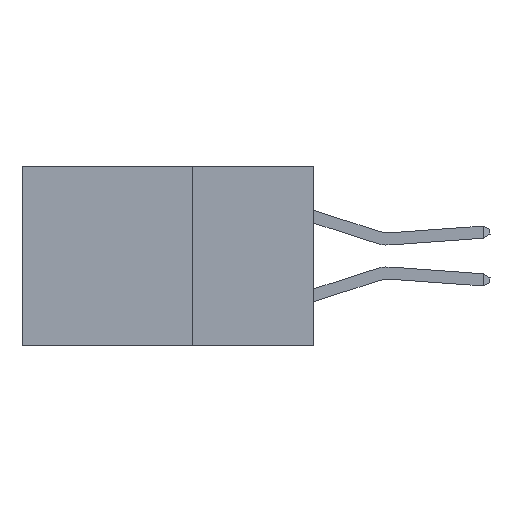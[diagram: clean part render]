
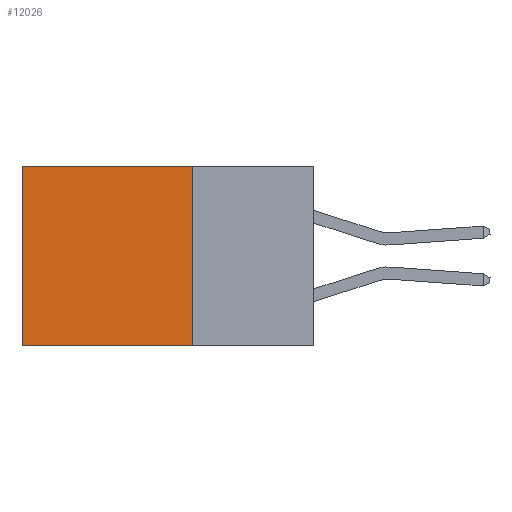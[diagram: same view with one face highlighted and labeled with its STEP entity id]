
A CAD part, left-side view. The second image highlights one B-rep face of the part: STEP entity #12026.
In plain terms, the highlighted planar face has unit normal (-1, 0, 0).
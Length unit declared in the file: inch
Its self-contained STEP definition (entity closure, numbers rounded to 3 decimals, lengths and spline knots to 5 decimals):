
#648 = AXIS2_PLACEMENT_3D ( 'NONE', #25661, #12626, #22278 ) ;
#1149 = VECTOR ( 'NONE', #2713, 39.37008 ) ;
#1549 = VERTEX_POINT ( 'NONE', #24139 ) ;
#2001 = CARTESIAN_POINT ( 'NONE',  ( 0.2875, 0.25, -0.37 ) ) ;
#2713 = DIRECTION ( 'NONE',  ( 0., 0., -1. ) ) ;
#3283 = CARTESIAN_POINT ( 'NONE',  ( 0.2875, 0.6, 0. ) ) ;
#3468 = DIRECTION ( 'NONE',  ( 0., 1., 0. ) ) ;
#3616 = EDGE_CURVE ( 'NONE', #1549, #25692, #10830, .T. ) ;
#3945 = VERTEX_POINT ( 'NONE', #22671 ) ;
#3960 = PLANE ( 'NONE',  #648 ) ;
#3964 = ORIENTED_EDGE ( 'NONE', *, *, #16884, .F. ) ;
#6012 = DIRECTION ( 'NONE',  ( 0., 1., 0. ) ) ;
#7553 = DIRECTION ( 'NONE',  ( 0., 0., -1. ) ) ;
#8371 = LINE ( 'NONE', #25355, #23628 ) ;
#8991 = EDGE_LOOP ( 'NONE', ( #12165, #3964, #16511, #22000 ) ) ;
#10705 = CARTESIAN_POINT ( 'NONE',  ( 0.2875, 0.6, -0.37 ) ) ;
#10830 = LINE ( 'NONE', #3283, #15815 ) ;
#12026 = ADVANCED_FACE ( 'NONE', ( #14006 ), #3960, .F. ) ;
#12165 = ORIENTED_EDGE ( 'NONE', *, *, #3616, .T. ) ;
#12626 = DIRECTION ( 'NONE',  ( 1., 0., 0. ) ) ;
#14006 = FACE_OUTER_BOUND ( 'NONE', #8991, .T. ) ;
#14038 = VERTEX_POINT ( 'NONE', #24936 ) ;
#15815 = VECTOR ( 'NONE', #7553, 39.37008 ) ;
#16511 = ORIENTED_EDGE ( 'NONE', *, *, #18328, .F. ) ;
#16884 = EDGE_CURVE ( 'NONE', #14038, #25692, #19911, .T. ) ;
#17410 = EDGE_CURVE ( 'NONE', #3945, #1549, #8371, .T. ) ;
#18256 = LINE ( 'NONE', #22740, #1149 ) ;
#18328 = EDGE_CURVE ( 'NONE', #3945, #14038, #18256, .T. ) ;
#18659 = VECTOR ( 'NONE', #6012, 39.37008 ) ;
#19911 = LINE ( 'NONE', #2001, #18659 ) ;
#22000 = ORIENTED_EDGE ( 'NONE', *, *, #17410, .T. ) ;
#22278 = DIRECTION ( 'NONE',  ( 0., 0., -1. ) ) ;
#22671 = CARTESIAN_POINT ( 'NONE',  ( 0.2875, 0.25, 0. ) ) ;
#22740 = CARTESIAN_POINT ( 'NONE',  ( 0.2875, 0.25, 0. ) ) ;
#23628 = VECTOR ( 'NONE', #3468, 39.37008 ) ;
#24139 = CARTESIAN_POINT ( 'NONE',  ( 0.2875, 0.6, 0. ) ) ;
#24936 = CARTESIAN_POINT ( 'NONE',  ( 0.2875, 0.25, -0.37 ) ) ;
#25355 = CARTESIAN_POINT ( 'NONE',  ( 0.2875, 0.25, 0. ) ) ;
#25661 = CARTESIAN_POINT ( 'NONE',  ( 0.2875, 0.25, 0. ) ) ;
#25692 = VERTEX_POINT ( 'NONE', #10705 ) ;
